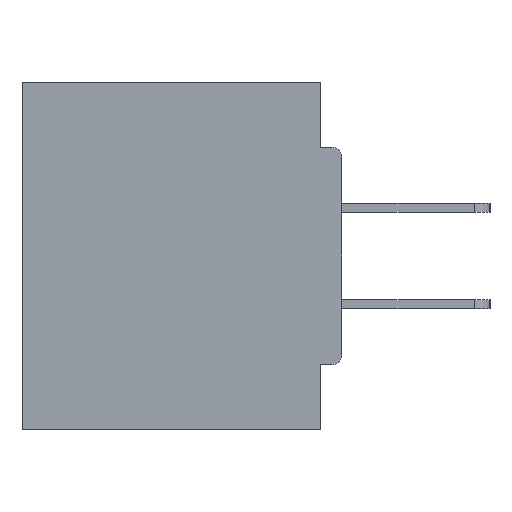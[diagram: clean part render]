
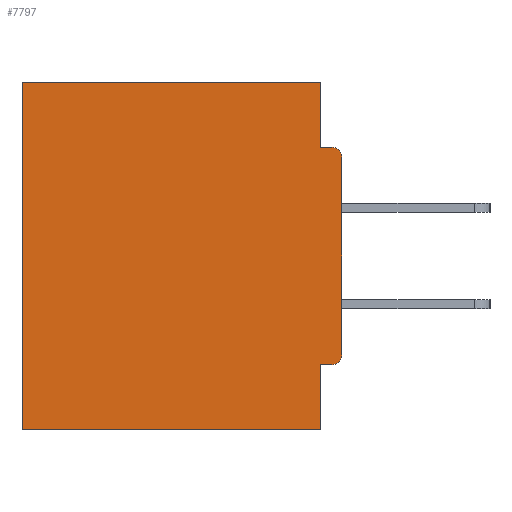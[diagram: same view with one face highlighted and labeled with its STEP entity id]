
A CAD part, left-side view. The second image highlights one B-rep face of the part: STEP entity #7797.
In plain terms, the highlighted planar face has unit normal (-1, 0, 0).
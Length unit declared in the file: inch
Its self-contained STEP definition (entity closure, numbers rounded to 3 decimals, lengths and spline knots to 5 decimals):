
#805 = VERTEX_POINT ( 'NONE', #1231 ) ;
#1231 = CARTESIAN_POINT ( 'NONE',  ( 0.298, 0.031, -0.0935 ) ) ;
#1460 = DIRECTION ( 'NONE',  ( 0., 0., -1. ) ) ;
#1753 = CARTESIAN_POINT ( 'NONE',  ( 0.298, 0., 0. ) ) ;
#2226 = VERTEX_POINT ( 'NONE', #25955 ) ;
#4034 = CARTESIAN_POINT ( 'NONE',  ( 0.298, 0., -0.1085 ) ) ;
#4554 = DIRECTION ( 'NONE',  ( 1., 0., 0. ) ) ;
#4769 = EDGE_CURVE ( 'NONE', #13154, #26155, #21521, .T. ) ;
#4900 = ORIENTED_EDGE ( 'NONE', *, *, #26345, .F. ) ;
#5034 = VECTOR ( 'NONE', #6225, 39.37008 ) ;
#5722 = VERTEX_POINT ( 'NONE', #22983 ) ;
#6225 = DIRECTION ( 'NONE',  ( 0., 0., -1. ) ) ;
#7100 = EDGE_CURVE ( 'NONE', #5722, #805, #9138, .T. ) ;
#7722 = LINE ( 'NONE', #11469, #37036 ) ;
#7797 = ADVANCED_FACE ( 'NONE', ( #21219 ), #10131, .F. ) ;
#7860 = CARTESIAN_POINT ( 'NONE',  ( 0.298, 0.015, -0.0935 ) ) ;
#9138 = LINE ( 'NONE', #30476, #25782 ) ;
#9184 = CARTESIAN_POINT ( 'NONE',  ( 0.298, 0., -0.0935 ) ) ;
#9481 = ORIENTED_EDGE ( 'NONE', *, *, #10483, .T. ) ;
#10131 = PLANE ( 'NONE',  #26365 ) ;
#10483 = EDGE_CURVE ( 'NONE', #34328, #32321, #12269, .T. ) ;
#11469 = CARTESIAN_POINT ( 'NONE',  ( 0.298, 0.031, -0.5 ) ) ;
#11541 = DIRECTION ( 'NONE',  ( 0., 1., 0. ) ) ;
#11616 = CIRCLE ( 'NONE', #24712, 0.015 ) ;
#11741 = ORIENTED_EDGE ( 'NONE', *, *, #19426, .F. ) ;
#11805 = CARTESIAN_POINT ( 'NONE',  ( 0.298, 0., 0. ) ) ;
#11886 = CARTESIAN_POINT ( 'NONE',  ( 0.298, 0.031, -0.4065 ) ) ;
#12269 = LINE ( 'NONE', #18518, #12742 ) ;
#12742 = VECTOR ( 'NONE', #33019, 39.37008 ) ;
#12987 = LINE ( 'NONE', #14324, #35078 ) ;
#13154 = VERTEX_POINT ( 'NONE', #4034 ) ;
#13304 = CARTESIAN_POINT ( 'NONE',  ( 0.298, 0.015, -0.3915 ) ) ;
#13995 = LINE ( 'NONE', #29024, #25243 ) ;
#14007 = EDGE_CURVE ( 'NONE', #15734, #23657, #24128, .T. ) ;
#14094 = DIRECTION ( 'NONE',  ( 0., 0., -1. ) ) ;
#14142 = EDGE_LOOP ( 'NONE', ( #29495, #36567, #27627, #14544, #9481, #11741, #4900, #28338, #27029, #20484 ) ) ;
#14324 = CARTESIAN_POINT ( 'NONE',  ( 0.298, 0., -0.5 ) ) ;
#14544 = ORIENTED_EDGE ( 'NONE', *, *, #17979, .T. ) ;
#15360 = CARTESIAN_POINT ( 'NONE',  ( 0.298, 0.46, 0. ) ) ;
#15734 = VERTEX_POINT ( 'NONE', #22720 ) ;
#15964 = DIRECTION ( 'NONE',  ( -1., 0., 0. ) ) ;
#16056 = VECTOR ( 'NONE', #31334, 39.37008 ) ;
#17979 = EDGE_CURVE ( 'NONE', #5722, #34328, #13995, .T. ) ;
#18518 = CARTESIAN_POINT ( 'NONE',  ( 0.298, 0.46, 0. ) ) ;
#19426 = EDGE_CURVE ( 'NONE', #2226, #32321, #12987, .T. ) ;
#20484 = ORIENTED_EDGE ( 'NONE', *, *, #25764, .F. ) ;
#20765 = DIRECTION ( 'NONE',  ( 0., -1., 0. ) ) ;
#21181 = CARTESIAN_POINT ( 'NONE',  ( 0.298, 0.46, -0.5 ) ) ;
#21219 = FACE_OUTER_BOUND ( 'NONE', #14142, .T. ) ;
#21521 = CIRCLE ( 'NONE', #32358, 0.015 ) ;
#21824 = EDGE_CURVE ( 'NONE', #15734, #23886, #11616, .T. ) ;
#22382 = CARTESIAN_POINT ( 'NONE',  ( 0.298, 0., -0.4065 ) ) ;
#22720 = CARTESIAN_POINT ( 'NONE',  ( 0.298, 0.015, -0.4065 ) ) ;
#22983 = CARTESIAN_POINT ( 'NONE',  ( 0.298, 0.031, 0. ) ) ;
#23657 = VERTEX_POINT ( 'NONE', #11886 ) ;
#23886 = VERTEX_POINT ( 'NONE', #30988 ) ;
#24128 = LINE ( 'NONE', #22382, #16056 ) ;
#24595 = VECTOR ( 'NONE', #20765, 39.37008 ) ;
#24712 = AXIS2_PLACEMENT_3D ( 'NONE', #13304, #24748, #36402 ) ;
#24748 = DIRECTION ( 'NONE',  ( -1., 0., 0. ) ) ;
#25243 = VECTOR ( 'NONE', #11541, 39.37008 ) ;
#25764 = EDGE_CURVE ( 'NONE', #13154, #23886, #30743, .T. ) ;
#25782 = VECTOR ( 'NONE', #14094, 39.37008 ) ;
#25955 = CARTESIAN_POINT ( 'NONE',  ( 0.298, 0.031, -0.5 ) ) ;
#26155 = VERTEX_POINT ( 'NONE', #7860 ) ;
#26345 = EDGE_CURVE ( 'NONE', #23657, #2226, #7722, .T. ) ;
#26365 = AXIS2_PLACEMENT_3D ( 'NONE', #1753, #4554, #30413 ) ;
#27029 = ORIENTED_EDGE ( 'NONE', *, *, #21824, .T. ) ;
#27627 = ORIENTED_EDGE ( 'NONE', *, *, #7100, .F. ) ;
#27639 = EDGE_CURVE ( 'NONE', #805, #26155, #31817, .T. ) ;
#28338 = ORIENTED_EDGE ( 'NONE', *, *, #14007, .F. ) ;
#28564 = DIRECTION ( 'NONE',  ( 0., 0., -1. ) ) ;
#29024 = CARTESIAN_POINT ( 'NONE',  ( 0.298, 0., 0. ) ) ;
#29495 = ORIENTED_EDGE ( 'NONE', *, *, #4769, .T. ) ;
#30413 = DIRECTION ( 'NONE',  ( 0., 0., -1. ) ) ;
#30476 = CARTESIAN_POINT ( 'NONE',  ( 0.298, 0.031, -0.5 ) ) ;
#30743 = LINE ( 'NONE', #11805, #5034 ) ;
#30988 = CARTESIAN_POINT ( 'NONE',  ( 0.298, 0., -0.3915 ) ) ;
#31334 = DIRECTION ( 'NONE',  ( 0., 1., 0. ) ) ;
#31817 = LINE ( 'NONE', #9184, #24595 ) ;
#32321 = VERTEX_POINT ( 'NONE', #21181 ) ;
#32358 = AXIS2_PLACEMENT_3D ( 'NONE', #33108, #15964, #1460 ) ;
#33019 = DIRECTION ( 'NONE',  ( 0., 0., -1. ) ) ;
#33108 = CARTESIAN_POINT ( 'NONE',  ( 0.298, 0.015, -0.1085 ) ) ;
#34328 = VERTEX_POINT ( 'NONE', #15360 ) ;
#34488 = DIRECTION ( 'NONE',  ( 0., 1., 0. ) ) ;
#35078 = VECTOR ( 'NONE', #34488, 39.37008 ) ;
#36402 = DIRECTION ( 'NONE',  ( 0., 0., -1. ) ) ;
#36567 = ORIENTED_EDGE ( 'NONE', *, *, #27639, .F. ) ;
#37036 = VECTOR ( 'NONE', #28564, 39.37008 ) ;
